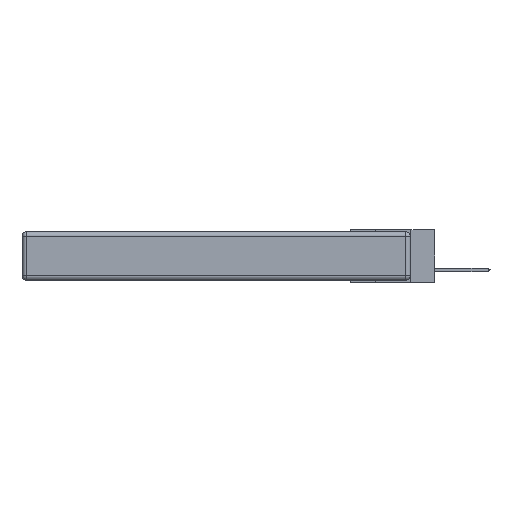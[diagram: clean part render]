
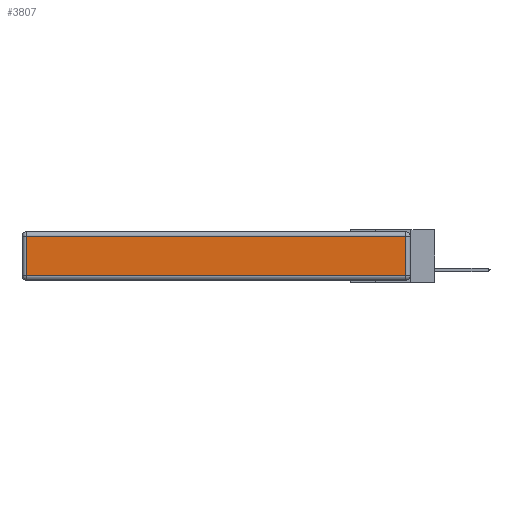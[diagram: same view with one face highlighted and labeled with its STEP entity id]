
A CAD part, left-side view. The second image highlights one B-rep face of the part: STEP entity #3807.
In plain terms, the highlighted planar face has unit normal (-1, 0, 0).
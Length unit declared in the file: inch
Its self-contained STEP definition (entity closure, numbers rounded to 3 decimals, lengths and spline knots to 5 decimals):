
#328 = VECTOR ( 'NONE', #1699, 39.37008 ) ;
#573 = EDGE_LOOP ( 'NONE', ( #14760, #9648, #5799, #7621 ) ) ;
#1699 = DIRECTION ( 'NONE',  ( 0., -1., 0. ) ) ;
#1962 = PLANE ( 'NONE',  #4624 ) ;
#2906 = CARTESIAN_POINT ( 'NONE',  ( 0., 0.03, -0.343 ) ) ;
#2940 = LINE ( 'NONE', #2906, #17399 ) ;
#3389 = DIRECTION ( 'NONE',  ( 0., 0., 1. ) ) ;
#3639 = DIRECTION ( 'NONE',  ( 0., 1., 0. ) ) ;
#3807 = ADVANCED_FACE ( 'NONE', ( #15947 ), #1962, .T. ) ;
#4114 = CARTESIAN_POINT ( 'NONE',  ( 0., 2.72, -0.03 ) ) ;
#4218 = EDGE_CURVE ( 'NONE', #13591, #13182, #9840, .T. ) ;
#4624 = AXIS2_PLACEMENT_3D ( 'NONE', #11764, #6356, #3389 ) ;
#5628 = DIRECTION ( 'NONE',  ( 0., 0., 1. ) ) ;
#5799 = ORIENTED_EDGE ( 'NONE', *, *, #4218, .T. ) ;
#6356 = DIRECTION ( 'NONE',  ( -1., 0., 0. ) ) ;
#7008 = VECTOR ( 'NONE', #3639, 39.37008 ) ;
#7346 = CARTESIAN_POINT ( 'NONE',  ( 0., 0.03, -0.03 ) ) ;
#7351 = VECTOR ( 'NONE', #15593, 39.37008 ) ;
#7621 = ORIENTED_EDGE ( 'NONE', *, *, #15261, .T. ) ;
#8135 = CARTESIAN_POINT ( 'NONE',  ( 0., 2.75, -0.03 ) ) ;
#8402 = CARTESIAN_POINT ( 'NONE',  ( 0., 2.72, -0.343 ) ) ;
#9648 = ORIENTED_EDGE ( 'NONE', *, *, #9911, .T. ) ;
#9840 = LINE ( 'NONE', #8135, #7008 ) ;
#9911 = EDGE_CURVE ( 'NONE', #16091, #13591, #2940, .T. ) ;
#10341 = CARTESIAN_POINT ( 'NONE',  ( 0., 0., -0.313 ) ) ;
#11415 = VERTEX_POINT ( 'NONE', #11442 ) ;
#11442 = CARTESIAN_POINT ( 'NONE',  ( 0., 2.72, -0.313 ) ) ;
#11764 = CARTESIAN_POINT ( 'NONE',  ( 0., 0., -0.343 ) ) ;
#13182 = VERTEX_POINT ( 'NONE', #4114 ) ;
#13591 = VERTEX_POINT ( 'NONE', #7346 ) ;
#13744 = EDGE_CURVE ( 'NONE', #11415, #16091, #17662, .T. ) ;
#14760 = ORIENTED_EDGE ( 'NONE', *, *, #13744, .T. ) ;
#15261 = EDGE_CURVE ( 'NONE', #13182, #11415, #16516, .T. ) ;
#15593 = DIRECTION ( 'NONE',  ( 0., 0., -1. ) ) ;
#15947 = FACE_OUTER_BOUND ( 'NONE', #573, .T. ) ;
#16091 = VERTEX_POINT ( 'NONE', #17463 ) ;
#16516 = LINE ( 'NONE', #8402, #7351 ) ;
#17399 = VECTOR ( 'NONE', #5628, 39.37008 ) ;
#17463 = CARTESIAN_POINT ( 'NONE',  ( 0., 0.03, -0.313 ) ) ;
#17662 = LINE ( 'NONE', #10341, #328 ) ;
